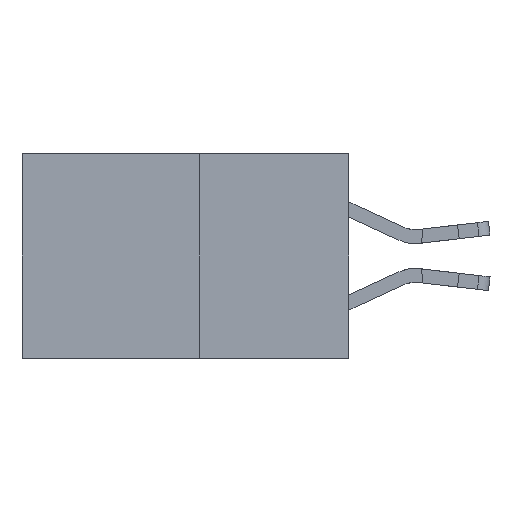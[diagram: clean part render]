
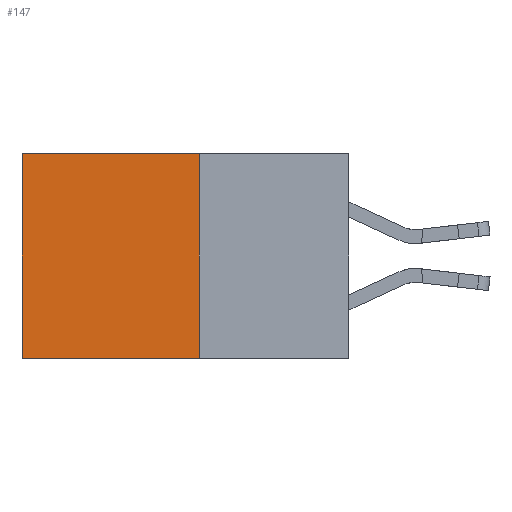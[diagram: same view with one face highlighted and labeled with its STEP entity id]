
A CAD part, left-side view. The second image highlights one B-rep face of the part: STEP entity #147.
In plain terms, the highlighted planar face has unit normal (-1, 0, 0).
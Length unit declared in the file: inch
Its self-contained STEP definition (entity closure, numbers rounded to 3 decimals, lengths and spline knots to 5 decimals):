
#147 = ADVANCED_FACE ( 'NONE', ( #18614 ), #10118, .F. ) ;
#1123 = VECTOR ( 'NONE', #13997, 39.37008 ) ;
#1432 = CARTESIAN_POINT ( 'NONE',  ( 0.277, 0.27, 0. ) ) ;
#1836 = ORIENTED_EDGE ( 'NONE', *, *, #8782, .T. ) ;
#2629 = EDGE_CURVE ( 'NONE', #10178, #5624, #4323, .T. ) ;
#4323 = LINE ( 'NONE', #5600, #11950 ) ;
#4922 = DIRECTION ( 'NONE',  ( 0., 1., 0. ) ) ;
#5196 = EDGE_CURVE ( 'NONE', #15935, #10178, #6774, .T. ) ;
#5600 = CARTESIAN_POINT ( 'NONE',  ( 0.277, 0.27, -0.37 ) ) ;
#5624 = VERTEX_POINT ( 'NONE', #18503 ) ;
#6714 = EDGE_CURVE ( 'NONE', #15935, #7205, #8851, .T. ) ;
#6734 = DIRECTION ( 'NONE',  ( 0., 0., -1. ) ) ;
#6774 = LINE ( 'NONE', #7556, #18385 ) ;
#7205 = VERTEX_POINT ( 'NONE', #19213 ) ;
#7542 = AXIS2_PLACEMENT_3D ( 'NONE', #9997, #13028, #10435 ) ;
#7556 = CARTESIAN_POINT ( 'NONE',  ( 0.277, 0.27, -0.37 ) ) ;
#7960 = CARTESIAN_POINT ( 'NONE',  ( 0.277, 0.27, -0.37 ) ) ;
#8782 = EDGE_CURVE ( 'NONE', #7205, #5624, #9259, .T. ) ;
#8851 = LINE ( 'NONE', #10354, #16479 ) ;
#9259 = LINE ( 'NONE', #12433, #1123 ) ;
#9997 = CARTESIAN_POINT ( 'NONE',  ( 0.277, 0.27, -0.37 ) ) ;
#10118 = PLANE ( 'NONE',  #7542 ) ;
#10178 = VERTEX_POINT ( 'NONE', #7960 ) ;
#10354 = CARTESIAN_POINT ( 'NONE',  ( 0.277, 0.27, 0. ) ) ;
#10435 = DIRECTION ( 'NONE',  ( 0., 0., -1. ) ) ;
#11152 = EDGE_LOOP ( 'NONE', ( #1836, #14777, #12234, #14757 ) ) ;
#11878 = DIRECTION ( 'NONE',  ( 0., 1., 0. ) ) ;
#11950 = VECTOR ( 'NONE', #4922, 39.37008 ) ;
#12234 = ORIENTED_EDGE ( 'NONE', *, *, #5196, .F. ) ;
#12433 = CARTESIAN_POINT ( 'NONE',  ( 0.277, 0.59, -0.37 ) ) ;
#13028 = DIRECTION ( 'NONE',  ( 1., 0., 0. ) ) ;
#13997 = DIRECTION ( 'NONE',  ( 0., 0., -1. ) ) ;
#14757 = ORIENTED_EDGE ( 'NONE', *, *, #6714, .T. ) ;
#14777 = ORIENTED_EDGE ( 'NONE', *, *, #2629, .F. ) ;
#15935 = VERTEX_POINT ( 'NONE', #1432 ) ;
#16479 = VECTOR ( 'NONE', #11878, 39.37008 ) ;
#18385 = VECTOR ( 'NONE', #6734, 39.37008 ) ;
#18503 = CARTESIAN_POINT ( 'NONE',  ( 0.277, 0.59, -0.37 ) ) ;
#18614 = FACE_OUTER_BOUND ( 'NONE', #11152, .T. ) ;
#19213 = CARTESIAN_POINT ( 'NONE',  ( 0.277, 0.59, 0. ) ) ;
